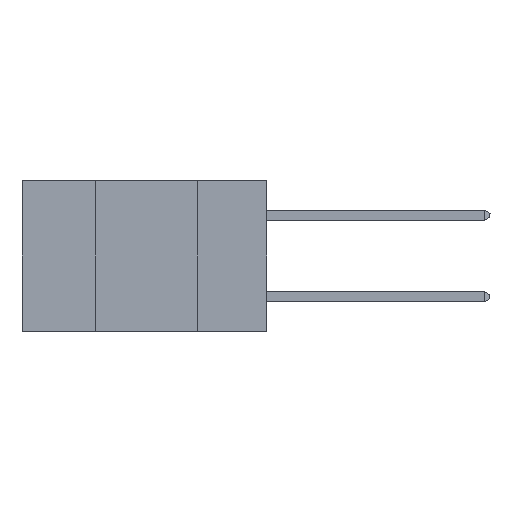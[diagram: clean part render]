
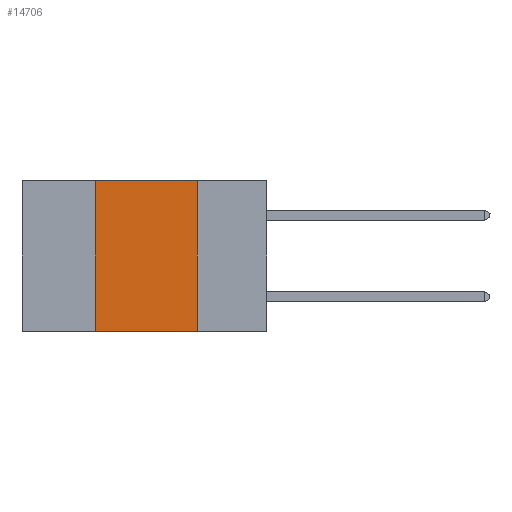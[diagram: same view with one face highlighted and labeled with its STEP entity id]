
A CAD part, left-side view. The second image highlights one B-rep face of the part: STEP entity #14706.
In plain terms, the highlighted planar face has unit normal (-1, 0, 0).
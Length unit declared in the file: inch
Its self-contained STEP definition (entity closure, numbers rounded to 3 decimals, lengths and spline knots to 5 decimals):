
#42 = EDGE_CURVE ( 'NONE', #23957, #14594, #7249, .T. ) ;
#1281 = CARTESIAN_POINT ( 'NONE',  ( 0., 0.17, 0. ) ) ;
#1603 = CARTESIAN_POINT ( 'NONE',  ( 0., 0.17, 0. ) ) ;
#2016 = DIRECTION ( 'NONE',  ( 1., 0., 0. ) ) ;
#3508 = ORIENTED_EDGE ( 'NONE', *, *, #12931, .F. ) ;
#3585 = CARTESIAN_POINT ( 'NONE',  ( 0., 0.6, -0.37 ) ) ;
#4824 = LINE ( 'NONE', #1281, #7817 ) ;
#5141 = DIRECTION ( 'NONE',  ( 0., 0., -1. ) ) ;
#7249 = LINE ( 'NONE', #15238, #21745 ) ;
#7449 = CARTESIAN_POINT ( 'NONE',  ( 0., 0.42, -0.37 ) ) ;
#7665 = LINE ( 'NONE', #19749, #9733 ) ;
#7817 = VECTOR ( 'NONE', #5141, 39.37008 ) ;
#8120 = CARTESIAN_POINT ( 'NONE',  ( 0., 0.17, -0.37 ) ) ;
#8319 = DIRECTION ( 'NONE',  ( 0., 0., 1. ) ) ;
#9723 = ORIENTED_EDGE ( 'NONE', *, *, #16586, .F. ) ;
#9733 = VECTOR ( 'NONE', #8319, 39.37008 ) ;
#11500 = LINE ( 'NONE', #3585, #16179 ) ;
#11623 = DIRECTION ( 'NONE',  ( 0., 0., -1. ) ) ;
#12931 = EDGE_CURVE ( 'NONE', #14594, #20402, #4824, .T. ) ;
#13288 = VERTEX_POINT ( 'NONE', #7449 ) ;
#14594 = VERTEX_POINT ( 'NONE', #1603 ) ;
#14706 = ADVANCED_FACE ( 'NONE', ( #16608 ), #20788, .F. ) ;
#15238 = CARTESIAN_POINT ( 'NONE',  ( 0., 0.6, 0. ) ) ;
#16179 = VECTOR ( 'NONE', #18769, 39.37008 ) ;
#16586 = EDGE_CURVE ( 'NONE', #13288, #23957, #7665, .T. ) ;
#16608 = FACE_OUTER_BOUND ( 'NONE', #16989, .T. ) ;
#16989 = EDGE_LOOP ( 'NONE', ( #3508, #20153, #9723, #21767 ) ) ;
#18769 = DIRECTION ( 'NONE',  ( 0., -1., 0. ) ) ;
#18989 = CARTESIAN_POINT ( 'NONE',  ( 0., 0.6, 0. ) ) ;
#19507 = CARTESIAN_POINT ( 'NONE',  ( 0., 0.42, 0. ) ) ;
#19749 = CARTESIAN_POINT ( 'NONE',  ( 0., 0.42, 0. ) ) ;
#20153 = ORIENTED_EDGE ( 'NONE', *, *, #42, .F. ) ;
#20402 = VERTEX_POINT ( 'NONE', #8120 ) ;
#20788 = PLANE ( 'NONE',  #20933 ) ;
#20933 = AXIS2_PLACEMENT_3D ( 'NONE', #18989, #2016, #11623 ) ;
#21745 = VECTOR ( 'NONE', #22857, 39.37008 ) ;
#21767 = ORIENTED_EDGE ( 'NONE', *, *, #23779, .T. ) ;
#22857 = DIRECTION ( 'NONE',  ( 0., -1., 0. ) ) ;
#23779 = EDGE_CURVE ( 'NONE', #13288, #20402, #11500, .T. ) ;
#23957 = VERTEX_POINT ( 'NONE', #19507 ) ;
